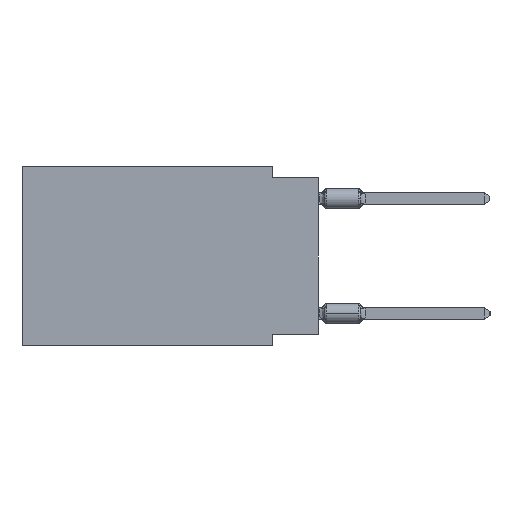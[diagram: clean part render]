
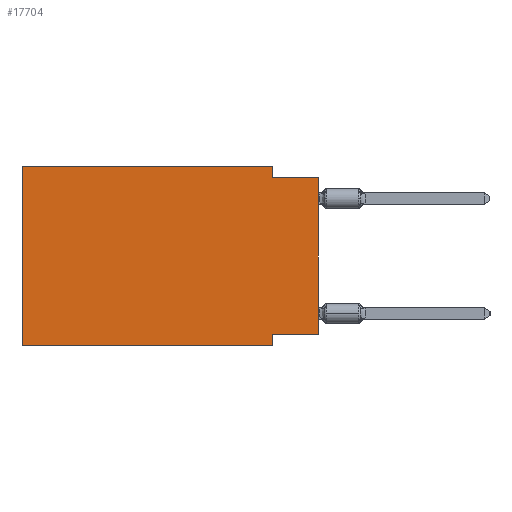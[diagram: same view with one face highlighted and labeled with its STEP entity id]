
A CAD part, left-side view. The second image highlights one B-rep face of the part: STEP entity #17704.
In plain terms, the highlighted planar face has unit normal (-1, 0, 0).
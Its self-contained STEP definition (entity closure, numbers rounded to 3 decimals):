
#284 = CARTESIAN_POINT ( 'NONE',  ( 0., 16.383, 0. ) ) ;
#1237 = VECTOR ( 'NONE', #11481, 1000. ) ;
#1905 = VERTEX_POINT ( 'NONE', #25136 ) ;
#2119 = EDGE_CURVE ( 'NONE', #3180, #14227, #21003, .T. ) ;
#2385 = DIRECTION ( 'NONE',  ( 0., -1., 0. ) ) ;
#2484 = ORIENTED_EDGE ( 'NONE', *, *, #2494, .F. ) ;
#2494 = EDGE_CURVE ( 'NONE', #14227, #18156, #9447, .T. ) ;
#2529 = LINE ( 'NONE', #21752, #4522 ) ;
#2641 = EDGE_CURVE ( 'NONE', #24223, #11177, #2529, .T. ) ;
#3118 = CARTESIAN_POINT ( 'NONE',  ( 0., 0., -9.271 ) ) ;
#3180 = VERTEX_POINT ( 'NONE', #3118 ) ;
#3516 = VECTOR ( 'NONE', #9020, 1000. ) ;
#3533 = VECTOR ( 'NONE', #2385, 1000. ) ;
#3642 = VERTEX_POINT ( 'NONE', #8827 ) ;
#3686 = CARTESIAN_POINT ( 'NONE',  ( 0., 16.383, -9.906 ) ) ;
#4128 = DIRECTION ( 'NONE',  ( 1., 0., 0. ) ) ;
#4522 = VECTOR ( 'NONE', #5362, 1000. ) ;
#5362 = DIRECTION ( 'NONE',  ( 0., 0., 1. ) ) ;
#6168 = FACE_OUTER_BOUND ( 'NONE', #31103, .T. ) ;
#7084 = DIRECTION ( 'NONE',  ( 0., 0., -1. ) ) ;
#8019 = VECTOR ( 'NONE', #17490, 1000. ) ;
#8101 = EDGE_CURVE ( 'NONE', #3180, #18931, #12898, .T. ) ;
#8827 = CARTESIAN_POINT ( 'NONE',  ( 0., 2.54, 0. ) ) ;
#8902 = ORIENTED_EDGE ( 'NONE', *, *, #2641, .F. ) ;
#9020 = DIRECTION ( 'NONE',  ( 0., 1., 0. ) ) ;
#9447 = LINE ( 'NONE', #20804, #25684 ) ;
#10164 = ORIENTED_EDGE ( 'NONE', *, *, #2119, .F. ) ;
#10386 = CARTESIAN_POINT ( 'NONE',  ( 0., 16.383, -9.906 ) ) ;
#11124 = EDGE_CURVE ( 'NONE', #3642, #1905, #16815, .T. ) ;
#11177 = VERTEX_POINT ( 'NONE', #284 ) ;
#11481 = DIRECTION ( 'NONE',  ( 0., 0., -1. ) ) ;
#12596 = LINE ( 'NONE', #10386, #20565 ) ;
#12803 = VECTOR ( 'NONE', #17170, 1000. ) ;
#12898 = LINE ( 'NONE', #20151, #12803 ) ;
#12947 = CARTESIAN_POINT ( 'NONE',  ( 0., 0., -0.635 ) ) ;
#13105 = ORIENTED_EDGE ( 'NONE', *, *, #17995, .T. ) ;
#13674 = CARTESIAN_POINT ( 'NONE',  ( 0., 2.54, -9.906 ) ) ;
#13711 = DIRECTION ( 'NONE',  ( 0., 0., -1. ) ) ;
#13727 = ORIENTED_EDGE ( 'NONE', *, *, #8101, .T. ) ;
#14227 = VERTEX_POINT ( 'NONE', #30141 ) ;
#14453 = CARTESIAN_POINT ( 'NONE',  ( 0., 2.54, 0. ) ) ;
#15757 = PLANE ( 'NONE',  #25621 ) ;
#16815 = LINE ( 'NONE', #14453, #1237 ) ;
#17170 = DIRECTION ( 'NONE',  ( 0., 0., 1. ) ) ;
#17490 = DIRECTION ( 'NONE',  ( 0., -1., 0. ) ) ;
#17704 = ADVANCED_FACE ( 'NONE', ( #6168 ), #15757, .F. ) ;
#17995 = EDGE_CURVE ( 'NONE', #24223, #18156, #12596, .T. ) ;
#18156 = VERTEX_POINT ( 'NONE', #13674 ) ;
#18931 = VERTEX_POINT ( 'NONE', #12947 ) ;
#19128 = EDGE_CURVE ( 'NONE', #11177, #3642, #28883, .T. ) ;
#19541 = CARTESIAN_POINT ( 'NONE',  ( 0., 16.383, 0. ) ) ;
#20151 = CARTESIAN_POINT ( 'NONE',  ( 0., 0., 0. ) ) ;
#20565 = VECTOR ( 'NONE', #29502, 1000. ) ;
#20804 = CARTESIAN_POINT ( 'NONE',  ( 0., 2.54, -9.906 ) ) ;
#21003 = LINE ( 'NONE', #30809, #3516 ) ;
#21032 = ORIENTED_EDGE ( 'NONE', *, *, #19128, .F. ) ;
#21752 = CARTESIAN_POINT ( 'NONE',  ( 0., 16.383, 0. ) ) ;
#22137 = EDGE_CURVE ( 'NONE', #1905, #18931, #24135, .T. ) ;
#23979 = CARTESIAN_POINT ( 'NONE',  ( 0., 0., -0.635 ) ) ;
#24135 = LINE ( 'NONE', #23979, #3533 ) ;
#24223 = VERTEX_POINT ( 'NONE', #3686 ) ;
#25136 = CARTESIAN_POINT ( 'NONE',  ( 0., 2.54, -0.635 ) ) ;
#25415 = CARTESIAN_POINT ( 'NONE',  ( 0., 16.383, 0. ) ) ;
#25621 = AXIS2_PLACEMENT_3D ( 'NONE', #25415, #4128, #13711 ) ;
#25684 = VECTOR ( 'NONE', #7084, 1000. ) ;
#26764 = ORIENTED_EDGE ( 'NONE', *, *, #11124, .F. ) ;
#28883 = LINE ( 'NONE', #19541, #8019 ) ;
#29502 = DIRECTION ( 'NONE',  ( 0., -1., 0. ) ) ;
#30141 = CARTESIAN_POINT ( 'NONE',  ( 0., 2.54, -9.271 ) ) ;
#30809 = CARTESIAN_POINT ( 'NONE',  ( 0., 0., -9.271 ) ) ;
#30860 = ORIENTED_EDGE ( 'NONE', *, *, #22137, .F. ) ;
#31103 = EDGE_LOOP ( 'NONE', ( #13727, #30860, #26764, #21032, #8902, #13105, #2484, #10164 ) ) ;
